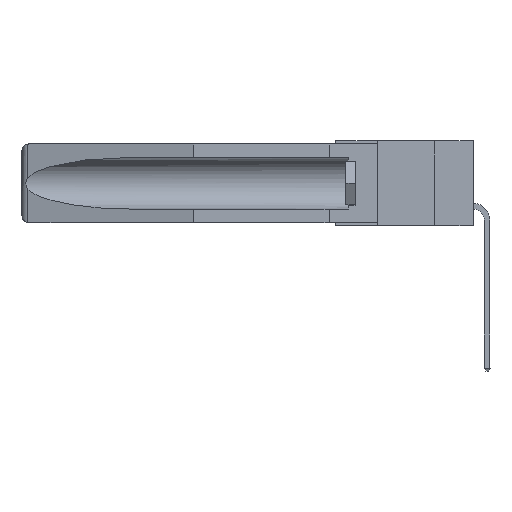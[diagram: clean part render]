
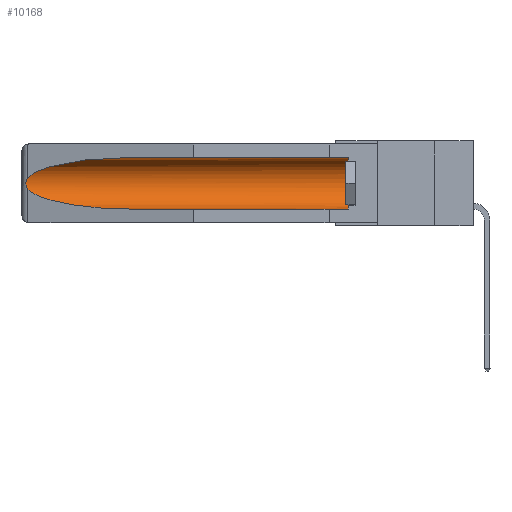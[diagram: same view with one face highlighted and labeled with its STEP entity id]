
A CAD part, left-side view. The second image highlights one B-rep face of the part: STEP entity #10168.
In plain terms, the highlighted cylindrical face has radius 2.857 mm (diameter 5.715 mm), a partial arc.
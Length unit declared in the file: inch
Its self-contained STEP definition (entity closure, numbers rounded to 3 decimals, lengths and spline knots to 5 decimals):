
#785 = ORIENTED_EDGE ( 'NONE', *, *, #22576, .F. ) ;
#1516 = CARTESIAN_POINT ( 'NONE',  ( 0.155, 0.126, -0.1715 ) ) ;
#1667 = CARTESIAN_POINT ( 'NONE',  ( 0.21114, 1.30732, -0.059 ) ) ;
#1844 = CARTESIAN_POINT ( 'NONE',  ( 0.155, 0.126, -0.059 ) ) ;
#2097 = CARTESIAN_POINT ( 'NONE',  ( 0.2675, 1.53308, -0.16763 ) ) ;
#2817 = DIRECTION ( 'NONE',  ( 0., 0., 1. ) ) ;
#2843 = EDGE_CURVE ( 'NONE', #7770, #15886, #22079, .T. ) ;
#3760 = DIRECTION ( 'NONE',  ( 0., 0., 1. ) ) ;
#4150 = CARTESIAN_POINT ( 'NONE',  ( 0.26597, 1.5296, -0.19026 ) ) ;
#4293 = VECTOR ( 'NONE', #26527, 39.37008 ) ;
#5388 = ORIENTED_EDGE ( 'NONE', *, *, #2843, .T. ) ;
#5797 = DIRECTION ( 'NONE',  ( 0., -1., 0. ) ) ;
#6015 = CARTESIAN_POINT ( 'NONE',  ( 0.2673, 1.53269, -0.17917 ) ) ;
#7770 = VERTEX_POINT ( 'NONE', #24364 ) ;
#7914 = CARTESIAN_POINT ( 'NONE',  ( 0.26537, 1.52718, -0.14972 ) ) ;
#7993 = CARTESIAN_POINT ( 'NONE',  ( 0.26597, 1.52961, -0.15275 ) ) ;
#8109 = CARTESIAN_POINT ( 'NONE',  ( 0.155, -0.30754, -0.284 ) ) ;
#9996 = EDGE_CURVE ( 'NONE', #13754, #19315, #18403, .T. ) ;
#10168 = ADVANCED_FACE ( 'NONE', ( #23002 ), #22338, .F. ) ;
#10352 = LINE ( 'NONE', #8109, #4293 ) ;
#11830 = CARTESIAN_POINT ( 'NONE',  ( 0.155, 1.07973, -0.059 ) ) ;
#12329 = CARTESIAN_POINT ( 'NONE',  ( 0.26537, 1.52718, -0.19328 ) ) ;
#12411 = ORIENTED_EDGE ( 'NONE', *, *, #22784, .T. ) ;
#12616 = CARTESIAN_POINT ( 'NONE',  ( 0.155, 1.07973, -0.284 ) ) ;
#13754 = VERTEX_POINT ( 'NONE', #15017 ) ;
#14137 = CARTESIAN_POINT ( 'NONE',  ( 0.21114, 1.30732, -0.284 ) ) ;
#14266 = CARTESIAN_POINT ( 'NONE',  ( 0.26537, 1.52718, -0.19328 ) ) ;
#14342 = CARTESIAN_POINT ( 'NONE',  ( 0.26654, 1.53092, -0.15636 ) ) ;
#14509 = ORIENTED_EDGE ( 'NONE', *, *, #21417, .T. ) ;
#14817 = B_SPLINE_CURVE_WITH_KNOTS ( 'NONE', 3,
 ( #24543, #7993, #14342, #20154, #2097, #16401, #6015, #16036, #4150, #14266 ),
 .UNSPECIFIED., .F., .F.,
 ( 4, 2, 2, 2, 4 ),
 ( 0., 0.00029, 0.00058, 0.00087, 0.00117 ),
 .UNSPECIFIED. ) ;
#14920 = VERTEX_POINT ( 'NONE', #19688 ) ;
#15017 = CARTESIAN_POINT ( 'NONE',  ( 0.26537, 1.52718, -0.19328 ) ) ;
#15303 = CARTESIAN_POINT ( 'NONE',  ( 0.155, 1.07973, -0.059 ) ) ;
#15491 = EDGE_LOOP ( 'NONE', ( #20295, #14509, #16599, #785, #5388, #12411 ) ) ;
#15886 = VERTEX_POINT ( 'NONE', #1844 ) ;
#16036 = CARTESIAN_POINT ( 'NONE',  ( 0.26655, 1.53094, -0.18657 ) ) ;
#16401 = CARTESIAN_POINT ( 'NONE',  ( 0.2675, 1.53308, -0.17534 ) ) ;
#16599 = ORIENTED_EDGE ( 'NONE', *, *, #9996, .T. ) ;
#18403 =( BOUNDED_CURVE ( )  B_SPLINE_CURVE ( 3, ( #12329, #18479, #14137, #20698 ),
 .UNSPECIFIED., .F., .F. ) 
 B_SPLINE_CURVE_WITH_KNOTS ( ( 4, 4 ),
 ( 0.1948, 1.5708 ),
 .UNSPECIFIED. ) 
 CURVE ( )  GEOMETRIC_REPRESENTATION_ITEM ( )  RATIONAL_B_SPLINE_CURVE ( ( 1., 0.848, 0.848, 1. ) ) 
 REPRESENTATION_ITEM ( '' )  );
#18422 = EDGE_CURVE ( 'NONE', #25424, #14920, #24328, .T. ) ;
#18479 = CARTESIAN_POINT ( 'NONE',  ( 0.25451, 1.48313, -0.24835 ) ) ;
#19004 = DIRECTION ( 'NONE',  ( 0., 1., 0. ) ) ;
#19315 = VERTEX_POINT ( 'NONE', #12616 ) ;
#19688 = CARTESIAN_POINT ( 'NONE',  ( 0.26537, 1.52718, -0.14972 ) ) ;
#20075 = CARTESIAN_POINT ( 'NONE',  ( 0.25451, 1.48313, -0.09465 ) ) ;
#20154 = CARTESIAN_POINT ( 'NONE',  ( 0.2673, 1.5327, -0.16383 ) ) ;
#20295 = ORIENTED_EDGE ( 'NONE', *, *, #18422, .T. ) ;
#20611 = AXIS2_PLACEMENT_3D ( 'NONE', #23043, #25242, #2817 ) ;
#20698 = CARTESIAN_POINT ( 'NONE',  ( 0.155, 1.07973, -0.284 ) ) ;
#21410 = CARTESIAN_POINT ( 'NONE',  ( 0.155, -0.30754, -0.059 ) ) ;
#21417 = EDGE_CURVE ( 'NONE', #14920, #13754, #14817, .T. ) ;
#22079 = CIRCLE ( 'NONE', #25985, 0.1125 ) ;
#22179 = LINE ( 'NONE', #21410, #25367 ) ;
#22338 = CYLINDRICAL_SURFACE ( 'NONE', #20611, 0.1125 ) ;
#22576 = EDGE_CURVE ( 'NONE', #7770, #19315, #10352, .T. ) ;
#22784 = EDGE_CURVE ( 'NONE', #15886, #25424, #22179, .T. ) ;
#23002 = FACE_OUTER_BOUND ( 'NONE', #15491, .T. ) ;
#23043 = CARTESIAN_POINT ( 'NONE',  ( 0.155, -0.30754, -0.1715 ) ) ;
#24328 =( BOUNDED_CURVE ( )  B_SPLINE_CURVE ( 3, ( #11830, #1667, #20075, #7914 ),
 .UNSPECIFIED., .F., .F. ) 
 B_SPLINE_CURVE_WITH_KNOTS ( ( 4, 4 ),
 ( 4.71239, 6.08839 ),
 .UNSPECIFIED. ) 
 CURVE ( )  GEOMETRIC_REPRESENTATION_ITEM ( )  RATIONAL_B_SPLINE_CURVE ( ( 1., 0.848, 0.848, 1. ) ) 
 REPRESENTATION_ITEM ( '' )  );
#24364 = CARTESIAN_POINT ( 'NONE',  ( 0.155, 0.126, -0.284 ) ) ;
#24543 = CARTESIAN_POINT ( 'NONE',  ( 0.26537, 1.52718, -0.14972 ) ) ;
#25242 = DIRECTION ( 'NONE',  ( 0., 1., 0. ) ) ;
#25367 = VECTOR ( 'NONE', #19004, 39.37008 ) ;
#25424 = VERTEX_POINT ( 'NONE', #15303 ) ;
#25985 = AXIS2_PLACEMENT_3D ( 'NONE', #1516, #5797, #3760 ) ;
#26527 = DIRECTION ( 'NONE',  ( 0., 1., 0. ) ) ;
